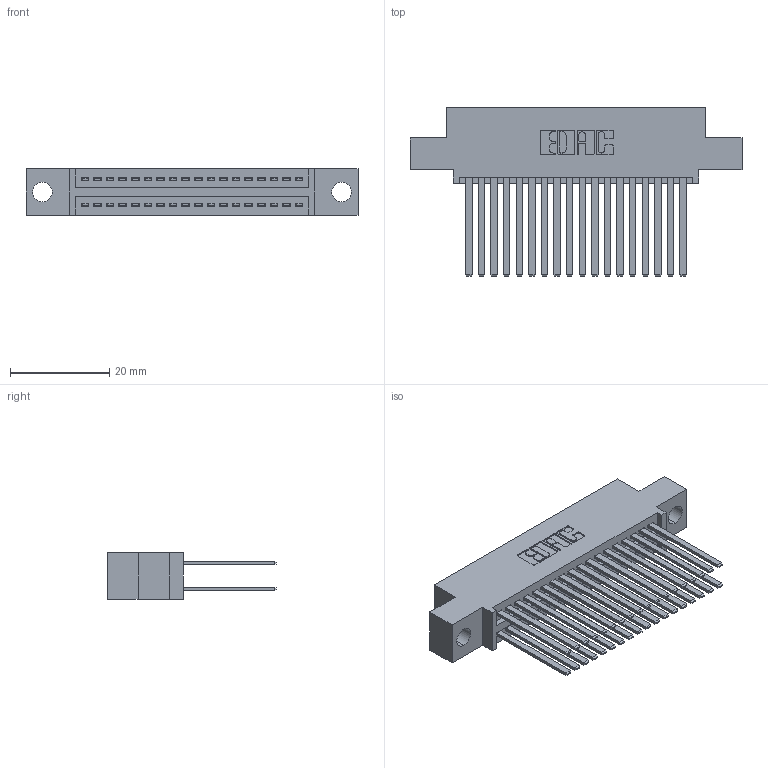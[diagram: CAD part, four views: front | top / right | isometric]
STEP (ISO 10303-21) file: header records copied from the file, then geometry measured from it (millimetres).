
FILE_DESCRIPTION (( 'STEP AP203' ), '1' );
FILE_NAME ('345-036-544-504.STEP', '2021-05-20T00:29:21', ( '' ), ( '' ), 'SwSTEP 2.0', 'SolidWorks 2020', '' );
FILE_SCHEMA (( 'CONFIG_CONTROL_DESIGN' ));
Length unit declared in the file: inch
Products named in the file (3): 345-036-544-504; 345-292-001_345-293-144; 345 Part_0.110 Offset - 0.156 Dia-TI
Assembly tree (37 placements, depth 2):
  345-036-544-504
    345 Part_0.110 Offset - 0.156 Dia-TI
    345-292-001_345-293-144  x36
Bounding box: 66.93 x 33.96 x 9.4 mm (x, y, z)
Volume: 6604.1 mm3; surface area: 10720.7 mm2
Topology: 37 solids, 37 shells, 1728 faces, 5105 edges, 3354 vertices
Faces by surface type: plane 1142, cylinder 586
Entity records: 17721 total; most frequent: CARTESIAN_POINT 2998, ORIENTED_EDGE 2930, DIRECTION 2669, EDGE_CURVE 1465, VECTOR 1265, LINE 1265, VERTEX_POINT 974, AXIS2_PLACEMENT_3D 702
